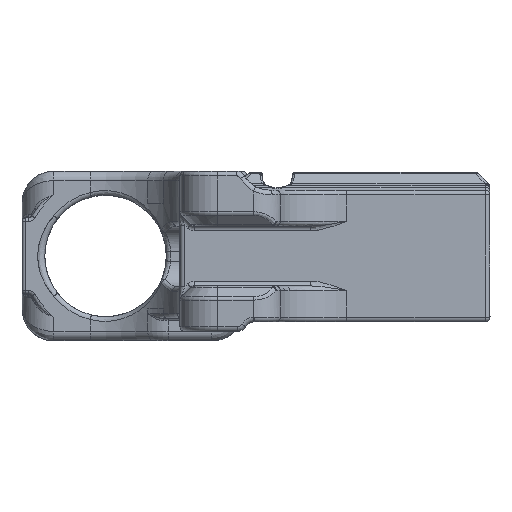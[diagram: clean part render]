
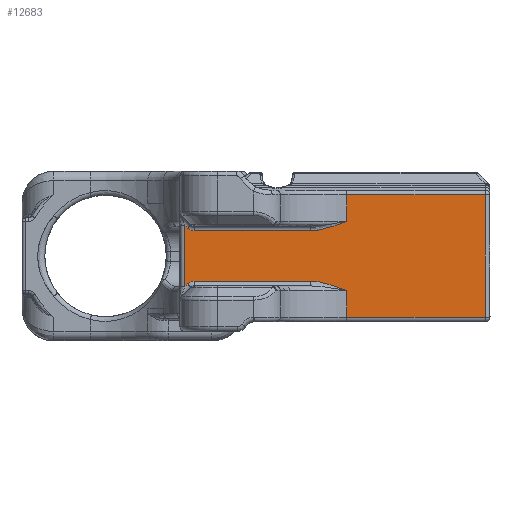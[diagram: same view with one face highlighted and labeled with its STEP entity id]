
A CAD part, left-side view. The second image highlights one B-rep face of the part: STEP entity #12683.
In plain terms, the highlighted planar face has unit normal (-1, 0, 0).
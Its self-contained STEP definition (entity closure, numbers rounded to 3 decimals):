
#140=PLANE('',#13623);
#644=CIRCLE('',#13462,2.);
#662=CIRCLE('',#13493,2.);
#1568=LINE('',#20088,#2356);
#1572=LINE('',#20241,#2360);
#1579=LINE('',#20361,#2367);
#1581=LINE('',#20364,#2369);
#1585=LINE('',#20373,#2373);
#1650=LINE('',#20728,#2438);
#1666=LINE('',#20839,#2454);
#1667=LINE('',#20841,#2455);
#1668=LINE('',#20843,#2456);
#1669=LINE('',#20844,#2457);
#2356=VECTOR('',#14970,10.);
#2360=VECTOR('',#14996,10.);
#2367=VECTOR('',#15039,10.);
#2369=VECTOR('',#15043,10.);
#2373=VECTOR('',#15053,10.);
#2438=VECTOR('',#15302,10.);
#2454=VECTOR('',#15380,10.);
#2455=VECTOR('',#15381,10.);
#2456=VECTOR('',#15382,10.);
#2457=VECTOR('',#15383,10.);
#3205=FACE_OUTER_BOUND('',#4035,.T.);
#4035=EDGE_LOOP('',(#8822,#8823,#8824,#8825,#8826,#8827,#8828,#8829,#8830,
#8831,#8832,#8833,#8834,#8835));
#4855=B_SPLINE_CURVE_WITH_KNOTS('',3,(#20130,#20131,#20132,#20133,#20134,
#20135,#20136,#20137),.UNSPECIFIED.,.F.,.F.,(4,1,1,2,4),(-0.791,
-0.316,-0.158,0.,0.001),
 .UNSPECIFIED.);
#4859=B_SPLINE_CURVE_WITH_KNOTS('',3,(#20351,#20352,#20353,#20354,#20355,
#20356,#20357,#20358),.UNSPECIFIED.,.F.,.F.,(4,2,1,1,4),(-0.792,
-0.791,-0.474,-0.316,0.),
 .UNSPECIFIED.);
#5252=VERTEX_POINT('',#20075);
#5253=VERTEX_POINT('',#20076);
#5256=VERTEX_POINT('',#20084);
#5258=VERTEX_POINT('',#20129);
#5263=VERTEX_POINT('',#20185);
#5265=VERTEX_POINT('',#20215);
#5280=VERTEX_POINT('',#20294);
#5281=VERTEX_POINT('',#20296);
#5282=VERTEX_POINT('',#20339);
#5284=VERTEX_POINT('',#20342);
#5394=VERTEX_POINT('',#20726);
#5419=VERTEX_POINT('',#20838);
#5420=VERTEX_POINT('',#20840);
#5421=VERTEX_POINT('',#20842);
#6448=EDGE_CURVE('',#5252,#5253,#644,.T.);
#6454=EDGE_CURVE('',#5253,#5256,#1568,.T.);
#6455=EDGE_CURVE('',#5256,#5258,#4855,.T.);
#6470=EDGE_CURVE('',#5265,#5263,#1572,.T.);
#6486=EDGE_CURVE('',#5280,#5281,#662,.T.);
#6490=EDGE_CURVE('',#5284,#5282,#4859,.T.);
#6492=EDGE_CURVE('',#5282,#5280,#1579,.T.);
#6494=EDGE_CURVE('',#5281,#5265,#1581,.T.);
#6499=EDGE_CURVE('',#5263,#5252,#1585,.T.);
#6638=EDGE_CURVE('',#5394,#5284,#1650,.T.);
#6676=EDGE_CURVE('',#5419,#5394,#1666,.T.);
#6677=EDGE_CURVE('',#5420,#5419,#1667,.T.);
#6678=EDGE_CURVE('',#5421,#5420,#1668,.T.);
#6679=EDGE_CURVE('',#5258,#5421,#1669,.T.);
#8822=ORIENTED_EDGE('',*,*,#6490,.F.);
#8823=ORIENTED_EDGE('',*,*,#6638,.F.);
#8824=ORIENTED_EDGE('',*,*,#6676,.F.);
#8825=ORIENTED_EDGE('',*,*,#6677,.F.);
#8826=ORIENTED_EDGE('',*,*,#6678,.F.);
#8827=ORIENTED_EDGE('',*,*,#6679,.F.);
#8828=ORIENTED_EDGE('',*,*,#6455,.F.);
#8829=ORIENTED_EDGE('',*,*,#6454,.F.);
#8830=ORIENTED_EDGE('',*,*,#6448,.F.);
#8831=ORIENTED_EDGE('',*,*,#6499,.F.);
#8832=ORIENTED_EDGE('',*,*,#6470,.F.);
#8833=ORIENTED_EDGE('',*,*,#6494,.F.);
#8834=ORIENTED_EDGE('',*,*,#6486,.F.);
#8835=ORIENTED_EDGE('',*,*,#6492,.F.);
#12683=ADVANCED_FACE('',(#3205),#140,.F.);
#13462=AXIS2_PLACEMENT_3D('',#20077,#14957,#14958);
#13493=AXIS2_PLACEMENT_3D('',#20297,#15030,#15031);
#13623=AXIS2_PLACEMENT_3D('',#20837,#15378,#15379);
#14957=DIRECTION('center_axis',(-1.,0.,0.));
#14958=DIRECTION('ref_axis',(0.,0.383,-0.924));
#14970=DIRECTION('',(0.,-1.,0.));
#14996=DIRECTION('',(0.,0.,1.));
#15030=DIRECTION('center_axis',(-1.,0.,0.));
#15031=DIRECTION('ref_axis',(0.,0.383,0.924));
#15039=DIRECTION('',(0.,1.,0.));
#15043=DIRECTION('',(0.,0.707,-0.707));
#15053=DIRECTION('',(0.,-0.707,-0.707));
#15302=DIRECTION('',(0.,0.,1.));
#15378=DIRECTION('center_axis',(1.,0.,0.));
#15379=DIRECTION('ref_axis',(0.,0.,-1.));
#15380=DIRECTION('',(0.,1.,0.));
#15381=DIRECTION('',(0.,0.,-1.));
#15382=DIRECTION('',(0.,-1.,0.));
#15383=DIRECTION('',(0.,0.,1.));
#20075=CARTESIAN_POINT('',(-184.248,-1.6,-5.291));
#20076=CARTESIAN_POINT('',(-184.248,-3.014,-5.877));
#20077=CARTESIAN_POINT('Origin',(-184.248,-3.014,-3.877));
#20084=CARTESIAN_POINT('',(-184.248,-27.728,-5.877));
#20088=CARTESIAN_POINT('',(-184.248,-49.328,-5.877));
#20129=CARTESIAN_POINT('',(-184.248,-35.39,-3.877));
#20130=CARTESIAN_POINT('Ctrl Pts',(-184.248,-27.728,
-5.877));
#20131=CARTESIAN_POINT('Ctrl Pts',(-184.248,-29.309,
-5.877));
#20132=CARTESIAN_POINT('Ctrl Pts',(-184.248,-31.368,
-5.342));
#20133=CARTESIAN_POINT('Ctrl Pts',(-184.248,-33.891,
-4.453));
#20134=CARTESIAN_POINT('Ctrl Pts',(-184.248,-34.885,
-4.07));
#20135=CARTESIAN_POINT('Ctrl Pts',(-184.248,-35.382,
-3.88));
#20136=CARTESIAN_POINT('Ctrl Pts',(-184.248,-35.386,
-3.878));
#20137=CARTESIAN_POINT('Ctrl Pts',(-184.248,-35.39,-3.877));
#20185=CARTESIAN_POINT('',(-184.248,-1.,-4.691));
#20215=CARTESIAN_POINT('',(-184.248,-1.,-17.763));
#20241=CARTESIAN_POINT('',(-184.248,-1.,-19.225));
#20294=CARTESIAN_POINT('',(-184.248,-3.014,-16.577));
#20296=CARTESIAN_POINT('',(-184.248,-1.6,-17.163));
#20297=CARTESIAN_POINT('Origin',(-184.248,-3.014,-18.577));
#20339=CARTESIAN_POINT('',(-184.248,-27.728,-16.577));
#20342=CARTESIAN_POINT('',(-184.248,-35.39,-18.577));
#20351=CARTESIAN_POINT('Ctrl Pts',(-184.248,-35.39,-18.577));
#20352=CARTESIAN_POINT('Ctrl Pts',(-184.248,-35.386,
-18.575));
#20353=CARTESIAN_POINT('Ctrl Pts',(-184.248,-35.382,
-18.574));
#20354=CARTESIAN_POINT('Ctrl Pts',(-184.248,-34.393,
-18.195));
#20355=CARTESIAN_POINT('Ctrl Pts',(-184.248,-32.888,
-17.616));
#20356=CARTESIAN_POINT('Ctrl Pts',(-184.248,-30.338,
-16.854));
#20357=CARTESIAN_POINT('Ctrl Pts',(-184.248,-28.782,-16.577));
#20358=CARTESIAN_POINT('Ctrl Pts',(-184.248,-27.728,
-16.577));
#20361=CARTESIAN_POINT('',(-184.248,-21.878,-16.577));
#20364=CARTESIAN_POINT('',(-184.248,-10.281,-8.482));
#20373=CARTESIAN_POINT('',(-184.248,-10.281,-13.972));
#20726=CARTESIAN_POINT('',(-184.248,-35.39,-24.222));
#20728=CARTESIAN_POINT('',(-184.248,-35.39,-18.225));
#20837=CARTESIAN_POINT('Origin',(-184.248,-32.401,-11.227));
#20838=CARTESIAN_POINT('',(-184.248,-64.797,-24.222));
#20839=CARTESIAN_POINT('',(-184.248,-34.466,-24.222));
#20840=CARTESIAN_POINT('',(-184.248,-64.797,1.769));
#20841=CARTESIAN_POINT('',(-184.248,-64.797,-18.225));
#20842=CARTESIAN_POINT('',(-184.248,-35.39,1.769));
#20843=CARTESIAN_POINT('',(-184.248,-34.466,1.769));
#20844=CARTESIAN_POINT('',(-184.248,-35.39,-8.052));
